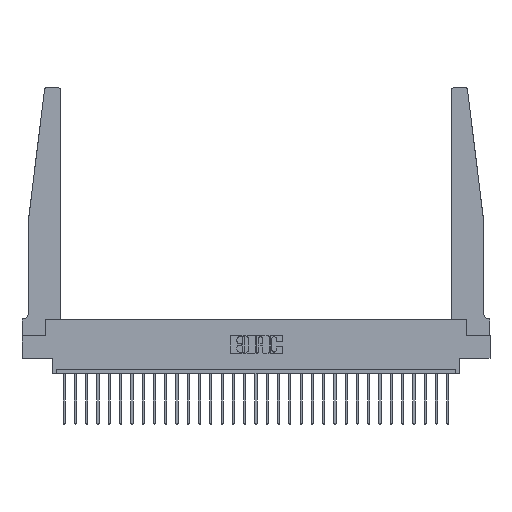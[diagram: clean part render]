
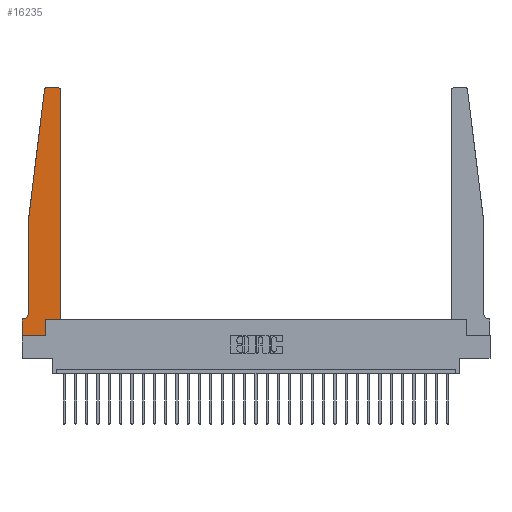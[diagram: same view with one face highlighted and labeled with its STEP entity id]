
A CAD part, top view. The second image highlights one B-rep face of the part: STEP entity #16235.
In plain terms, the highlighted planar face has unit normal (0, 0, 1).
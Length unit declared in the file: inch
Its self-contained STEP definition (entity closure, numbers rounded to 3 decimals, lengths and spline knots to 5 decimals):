
#5 = CARTESIAN_POINT ( 'NONE',  ( 0., 0.1875, 0.37 ) ) ;
#83 = DIRECTION ( 'NONE',  ( 1., 0., 0. ) ) ;
#481 = CARTESIAN_POINT ( 'NONE',  ( 0.065, 1.25, 0.37 ) ) ;
#523 = FACE_OUTER_BOUND ( 'NONE', #12429, .T. ) ;
#574 = DIRECTION ( 'NONE',  ( -1., 0., 0. ) ) ;
#620 = ORIENTED_EDGE ( 'NONE', *, *, #19192, .T. ) ;
#699 = ORIENTED_EDGE ( 'NONE', *, *, #18726, .T. ) ;
#971 = DIRECTION ( 'NONE',  ( 0., -1., 0. ) ) ;
#1079 = CARTESIAN_POINT ( 'NONE',  ( 0., 0.1875, 0.37 ) ) ;
#1877 = VERTEX_POINT ( 'NONE', #1079 ) ;
#2362 = VECTOR ( 'NONE', #7079, 39.37008 ) ;
#2803 = CARTESIAN_POINT ( 'NONE',  ( 0.425, 0.18, 0.37 ) ) ;
#3106 = CARTESIAN_POINT ( 'NONE',  ( 0., 0., 0.37 ) ) ;
#3204 = DIRECTION ( 'NONE',  ( 1., 0., 0. ) ) ;
#3679 = VERTEX_POINT ( 'NONE', #24365 ) ;
#3796 = CARTESIAN_POINT ( 'NONE',  ( 0.2605, 0.18, 0.37 ) ) ;
#4201 = EDGE_CURVE ( 'NONE', #15166, #21676, #24661, .T. ) ;
#4284 = LINE ( 'NONE', #21650, #9272 ) ;
#4654 = EDGE_CURVE ( 'NONE', #16460, #1877, #4284, .T. ) ;
#5039 = CARTESIAN_POINT ( 'NONE',  ( 0.425, 0.18, 0.37 ) ) ;
#5363 = CARTESIAN_POINT ( 'NONE',  ( 0.395, 2.72, 0.37 ) ) ;
#6261 = VERTEX_POINT ( 'NONE', #12995 ) ;
#7079 = DIRECTION ( 'NONE',  ( 0., -1., 0. ) ) ;
#7101 = DIRECTION ( 'NONE',  ( 1., 0., 0. ) ) ;
#7103 = VECTOR ( 'NONE', #3204, 39.37008 ) ;
#7315 = CARTESIAN_POINT ( 'NONE',  ( 0.27653, 2.75, 0.37 ) ) ;
#7800 = AXIS2_PLACEMENT_3D ( 'NONE', #8483, #23391, #12764 ) ;
#7924 = CARTESIAN_POINT ( 'NONE',  ( 0.395, 2.75, 0.37 ) ) ;
#8483 = CARTESIAN_POINT ( 'NONE',  ( 0.27653, 2.72, 0.37 ) ) ;
#8639 = EDGE_CURVE ( 'NONE', #17150, #27021, #25097, .T. ) ;
#8761 = EDGE_CURVE ( 'NONE', #24515, #6261, #13733, .T. ) ;
#9088 = CARTESIAN_POINT ( 'NONE',  ( 0.2605, 0.18, 0.37 ) ) ;
#9272 = VECTOR ( 'NONE', #574, 39.37008 ) ;
#9340 = CARTESIAN_POINT ( 'NONE',  ( 0.425, 2.72, 0.37 ) ) ;
#9592 = ORIENTED_EDGE ( 'NONE', *, *, #11164, .T. ) ;
#11164 = EDGE_CURVE ( 'NONE', #11807, #24752, #25408, .T. ) ;
#11293 = VECTOR ( 'NONE', #7101, 39.37008 ) ;
#11640 = CARTESIAN_POINT ( 'NONE',  ( 0.25, 2.75, 0.37 ) ) ;
#11807 = VERTEX_POINT ( 'NONE', #9340 ) ;
#11848 = ORIENTED_EDGE ( 'NONE', *, *, #21255, .T. ) ;
#12420 = EDGE_CURVE ( 'NONE', #1877, #24515, #21024, .T. ) ;
#12429 = EDGE_LOOP ( 'NONE', ( #620, #14172, #16651, #22305, #11848, #24667, #14196, #22452, #22043, #16898, #699, #9592 ) ) ;
#12493 = EDGE_CURVE ( 'NONE', #27021, #3679, #26372, .T. ) ;
#12595 = CARTESIAN_POINT ( 'NONE',  ( 0.015, 0.2375, 0.37 ) ) ;
#12764 = DIRECTION ( 'NONE',  ( 1., 0., 0. ) ) ;
#12995 = CARTESIAN_POINT ( 'NONE',  ( 0.2605, 0., 0.37 ) ) ;
#13273 = AXIS2_PLACEMENT_3D ( 'NONE', #5, #18671, #83 ) ;
#13633 = LINE ( 'NONE', #11640, #19620 ) ;
#13733 = LINE ( 'NONE', #3106, #7103 ) ;
#13775 = DIRECTION ( 'NONE',  ( -1., 0., 0. ) ) ;
#14010 = VECTOR ( 'NONE', #24410, 39.37008 ) ;
#14172 = ORIENTED_EDGE ( 'NONE', *, *, #20745, .T. ) ;
#14196 = ORIENTED_EDGE ( 'NONE', *, *, #12420, .T. ) ;
#14974 = AXIS2_PLACEMENT_3D ( 'NONE', #5363, #18194, #15686 ) ;
#15166 = VERTEX_POINT ( 'NONE', #3796 ) ;
#15460 = AXIS2_PLACEMENT_3D ( 'NONE', #12595, #18911, #23023 ) ;
#15686 = DIRECTION ( 'NONE',  ( 1., 0., 0. ) ) ;
#15718 = CARTESIAN_POINT ( 'NONE',  ( 0., 0., 0.37 ) ) ;
#16079 = CARTESIAN_POINT ( 'NONE',  ( 0.425, 0.18, 0.37 ) ) ;
#16235 = ADVANCED_FACE ( 'NONE', ( #523 ), #23181, .T. ) ;
#16396 = CARTESIAN_POINT ( 'NONE',  ( 0., 0., 0.37 ) ) ;
#16460 = VERTEX_POINT ( 'NONE', #19968 ) ;
#16651 = ORIENTED_EDGE ( 'NONE', *, *, #8639, .T. ) ;
#16898 = ORIENTED_EDGE ( 'NONE', *, *, #4201, .T. ) ;
#17062 = VECTOR ( 'NONE', #26307, 39.37008 ) ;
#17150 = VERTEX_POINT ( 'NONE', #24678 ) ;
#17886 = CIRCLE ( 'NONE', #15460, 0.05 ) ;
#18194 = DIRECTION ( 'NONE',  ( 0., 0., 1. ) ) ;
#18671 = DIRECTION ( 'NONE',  ( 0., 0., 1. ) ) ;
#18726 = EDGE_CURVE ( 'NONE', #21676, #11807, #19667, .T. ) ;
#18911 = DIRECTION ( 'NONE',  ( 0., 0., -1. ) ) ;
#19192 = EDGE_CURVE ( 'NONE', #24752, #22826, #13633, .T. ) ;
#19620 = VECTOR ( 'NONE', #13775, 39.37008 ) ;
#19667 = LINE ( 'NONE', #2803, #14010 ) ;
#19968 = CARTESIAN_POINT ( 'NONE',  ( 0.015, 0.1875, 0.37 ) ) ;
#20745 = EDGE_CURVE ( 'NONE', #22826, #17150, #23618, .T. ) ;
#21024 = LINE ( 'NONE', #15718, #25048 ) ;
#21255 = EDGE_CURVE ( 'NONE', #3679, #16460, #17886, .T. ) ;
#21650 = CARTESIAN_POINT ( 'NONE',  ( 0.065, 0.1875, 0.37 ) ) ;
#21676 = VERTEX_POINT ( 'NONE', #16079 ) ;
#22043 = ORIENTED_EDGE ( 'NONE', *, *, #22727, .T. ) ;
#22305 = ORIENTED_EDGE ( 'NONE', *, *, #12493, .T. ) ;
#22452 = ORIENTED_EDGE ( 'NONE', *, *, #8761, .T. ) ;
#22727 = EDGE_CURVE ( 'NONE', #6261, #15166, #26561, .T. ) ;
#22826 = VERTEX_POINT ( 'NONE', #7315 ) ;
#23023 = DIRECTION ( 'NONE',  ( -1., 0., 0. ) ) ;
#23181 = PLANE ( 'NONE',  #13273 ) ;
#23391 = DIRECTION ( 'NONE',  ( 0., 0., 1. ) ) ;
#23618 = CIRCLE ( 'NONE', #7800, 0.03 ) ;
#23989 = CARTESIAN_POINT ( 'NONE',  ( 0.065, 1.25, 0.37 ) ) ;
#24204 = CARTESIAN_POINT ( 'NONE',  ( 0.065, 1.25, 0.37 ) ) ;
#24365 = CARTESIAN_POINT ( 'NONE',  ( 0.065, 0.2375, 0.37 ) ) ;
#24410 = DIRECTION ( 'NONE',  ( 0., 1., 0. ) ) ;
#24515 = VERTEX_POINT ( 'NONE', #16396 ) ;
#24661 = LINE ( 'NONE', #5039, #11293 ) ;
#24667 = ORIENTED_EDGE ( 'NONE', *, *, #4654, .T. ) ;
#24678 = CARTESIAN_POINT ( 'NONE',  ( 0.24675, 2.72367, 0.37 ) ) ;
#24752 = VERTEX_POINT ( 'NONE', #7924 ) ;
#25048 = VECTOR ( 'NONE', #971, 39.37008 ) ;
#25097 = LINE ( 'NONE', #23989, #17062 ) ;
#25408 = CIRCLE ( 'NONE', #14974, 0.03 ) ;
#25903 = VECTOR ( 'NONE', #26156, 39.37008 ) ;
#26156 = DIRECTION ( 'NONE',  ( 0., 1., 0. ) ) ;
#26307 = DIRECTION ( 'NONE',  ( -0.122, -0.992, 0. ) ) ;
#26372 = LINE ( 'NONE', #481, #2362 ) ;
#26561 = LINE ( 'NONE', #9088, #25903 ) ;
#27021 = VERTEX_POINT ( 'NONE', #24204 ) ;
